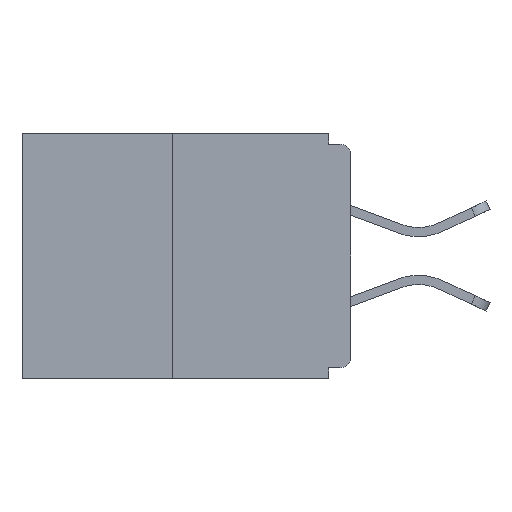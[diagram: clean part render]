
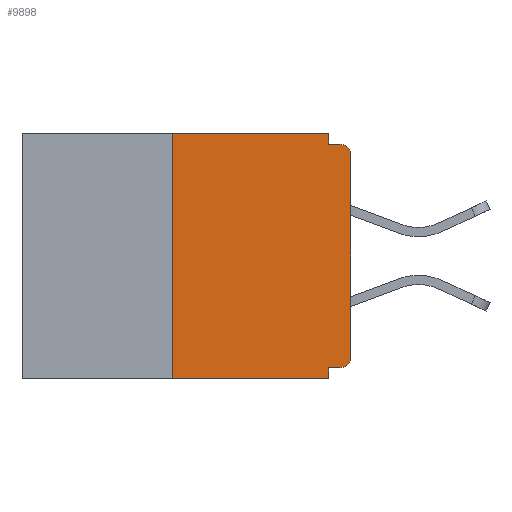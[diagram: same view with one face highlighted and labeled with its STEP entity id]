
A CAD part, left-side view. The second image highlights one B-rep face of the part: STEP entity #9898.
In plain terms, the highlighted planar face has unit normal (-1, 0, 0).
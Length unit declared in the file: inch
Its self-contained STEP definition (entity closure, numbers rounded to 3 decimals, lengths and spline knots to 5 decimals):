
#55 = DIRECTION ( 'NONE',  ( 0., 0., -1. ) ) ;
#77 = VERTEX_POINT ( 'NONE', #13116 ) ;
#89 = ORIENTED_EDGE ( 'NONE', *, *, #696, .F. ) ;
#140 = EDGE_CURVE ( 'NONE', #28373, #24476, #27689, .T. ) ;
#260 = CARTESIAN_POINT ( 'NONE',  ( 0., 0., 0. ) ) ;
#696 = EDGE_CURVE ( 'NONE', #29795, #15816, #27579, .T. ) ;
#936 = CARTESIAN_POINT ( 'NONE',  ( 0., 0.031, -0.343 ) ) ;
#1424 = CARTESIAN_POINT ( 'NONE',  ( 0., 0.015, -0.03 ) ) ;
#1528 = DIRECTION ( 'NONE',  ( 0., -1., 0. ) ) ;
#2436 = ORIENTED_EDGE ( 'NONE', *, *, #25723, .F. ) ;
#3128 = PLANE ( 'NONE',  #16647 ) ;
#3170 = CARTESIAN_POINT ( 'NONE',  ( 0., 0.031, 0. ) ) ;
#3340 = DIRECTION ( 'NONE',  ( 0., 0., -1. ) ) ;
#3561 = CARTESIAN_POINT ( 'NONE',  ( 0., 0., -0.313 ) ) ;
#3753 = CARTESIAN_POINT ( 'NONE',  ( 0., 0., -0.328 ) ) ;
#3880 = CARTESIAN_POINT ( 'NONE',  ( 0., 0., -0.03 ) ) ;
#3927 = CARTESIAN_POINT ( 'NONE',  ( 0., 0.031, 0. ) ) ;
#4766 = LINE ( 'NONE', #23429, #12398 ) ;
#4807 = ORIENTED_EDGE ( 'NONE', *, *, #20768, .T. ) ;
#4923 = VECTOR ( 'NONE', #12303, 39.37008 ) ;
#5707 = VECTOR ( 'NONE', #8784, 39.37008 ) ;
#6485 = LINE ( 'NONE', #13892, #5707 ) ;
#6752 = EDGE_CURVE ( 'NONE', #15816, #22791, #4766, .T. ) ;
#6961 = DIRECTION ( 'NONE',  ( -1., 0., 0. ) ) ;
#7391 = VERTEX_POINT ( 'NONE', #25448 ) ;
#7812 = LINE ( 'NONE', #260, #4923 ) ;
#7909 = CIRCLE ( 'NONE', #10279, 0.015 ) ;
#8032 = LINE ( 'NONE', #11750, #19474 ) ;
#8784 = DIRECTION ( 'NONE',  ( 0., 0., -1. ) ) ;
#9290 = ORIENTED_EDGE ( 'NONE', *, *, #6752, .F. ) ;
#9316 = ORIENTED_EDGE ( 'NONE', *, *, #140, .T. ) ;
#9734 = DIRECTION ( 'NONE',  ( 0., -1., 0. ) ) ;
#9898 = ADVANCED_FACE ( 'NONE', ( #25603 ), #3128, .F. ) ;
#10116 = EDGE_CURVE ( 'NONE', #22791, #7391, #23639, .T. ) ;
#10279 = AXIS2_PLACEMENT_3D ( 'NONE', #14534, #6961, #55 ) ;
#10282 = ORIENTED_EDGE ( 'NONE', *, *, #28740, .T. ) ;
#11229 = CARTESIAN_POINT ( 'NONE',  ( 0., 0.25, 0. ) ) ;
#11750 = CARTESIAN_POINT ( 'NONE',  ( 0., 0., -0.015 ) ) ;
#12006 = VECTOR ( 'NONE', #30299, 39.37008 ) ;
#12303 = DIRECTION ( 'NONE',  ( 0., 0., 1. ) ) ;
#12327 = LINE ( 'NONE', #28982, #19585 ) ;
#12398 = VECTOR ( 'NONE', #1528, 39.37008 ) ;
#12668 = EDGE_CURVE ( 'NONE', #7391, #24476, #8032, .T. ) ;
#13116 = CARTESIAN_POINT ( 'NONE',  ( 0., 0.031, -0.328 ) ) ;
#13540 = DIRECTION ( 'NONE',  ( 0., 0., -1. ) ) ;
#13892 = CARTESIAN_POINT ( 'NONE',  ( 0., 0.031, -0.343 ) ) ;
#14534 = CARTESIAN_POINT ( 'NONE',  ( 0., 0.015, -0.313 ) ) ;
#15384 = DIRECTION ( 'NONE',  ( 1., 0., 0. ) ) ;
#15688 = DIRECTION ( 'NONE',  ( -1., 0., 0. ) ) ;
#15816 = VERTEX_POINT ( 'NONE', #11229 ) ;
#16279 = VERTEX_POINT ( 'NONE', #3561 ) ;
#16340 = DIRECTION ( 'NONE',  ( 0., 1., 0. ) ) ;
#16647 = AXIS2_PLACEMENT_3D ( 'NONE', #27402, #15384, #3340 ) ;
#17050 = CARTESIAN_POINT ( 'NONE',  ( 0., 0.25, -0.343 ) ) ;
#17673 = VECTOR ( 'NONE', #16340, 39.37008 ) ;
#18310 = CARTESIAN_POINT ( 'NONE',  ( 0., 0.015, -0.015 ) ) ;
#18668 = ORIENTED_EDGE ( 'NONE', *, *, #10116, .F. ) ;
#19399 = AXIS2_PLACEMENT_3D ( 'NONE', #1424, #15688, #13540 ) ;
#19474 = VECTOR ( 'NONE', #23657, 39.37008 ) ;
#19585 = VECTOR ( 'NONE', #9734, 39.37008 ) ;
#19959 = LINE ( 'NONE', #3753, #17673 ) ;
#20010 = DIRECTION ( 'NONE',  ( 0., 0., -1. ) ) ;
#20768 = EDGE_CURVE ( 'NONE', #29795, #22190, #12327, .T. ) ;
#22190 = VERTEX_POINT ( 'NONE', #936 ) ;
#22227 = EDGE_LOOP ( 'NONE', ( #9290, #89, #4807, #25659, #2436, #26772, #10282, #9316, #24820, #18668 ) ) ;
#22791 = VERTEX_POINT ( 'NONE', #3927 ) ;
#23109 = CARTESIAN_POINT ( 'NONE',  ( 0., 0.25, 0. ) ) ;
#23429 = CARTESIAN_POINT ( 'NONE',  ( 0., 0.46, 0. ) ) ;
#23639 = LINE ( 'NONE', #3170, #28563 ) ;
#23657 = DIRECTION ( 'NONE',  ( 0., -1., 0. ) ) ;
#24476 = VERTEX_POINT ( 'NONE', #18310 ) ;
#24820 = ORIENTED_EDGE ( 'NONE', *, *, #12668, .F. ) ;
#25247 = CARTESIAN_POINT ( 'NONE',  ( 0., 0.015, -0.328 ) ) ;
#25448 = CARTESIAN_POINT ( 'NONE',  ( 0., 0.031, -0.015 ) ) ;
#25603 = FACE_OUTER_BOUND ( 'NONE', #22227, .T. ) ;
#25659 = ORIENTED_EDGE ( 'NONE', *, *, #28487, .F. ) ;
#25723 = EDGE_CURVE ( 'NONE', #31284, #77, #19959, .T. ) ;
#26772 = ORIENTED_EDGE ( 'NONE', *, *, #29206, .T. ) ;
#27402 = CARTESIAN_POINT ( 'NONE',  ( 0., 0.46, 0. ) ) ;
#27579 = LINE ( 'NONE', #23109, #12006 ) ;
#27689 = CIRCLE ( 'NONE', #19399, 0.015 ) ;
#28373 = VERTEX_POINT ( 'NONE', #3880 ) ;
#28487 = EDGE_CURVE ( 'NONE', #77, #22190, #6485, .T. ) ;
#28563 = VECTOR ( 'NONE', #20010, 39.37008 ) ;
#28740 = EDGE_CURVE ( 'NONE', #16279, #28373, #7812, .T. ) ;
#28982 = CARTESIAN_POINT ( 'NONE',  ( 0., 0.46, -0.343 ) ) ;
#29206 = EDGE_CURVE ( 'NONE', #31284, #16279, #7909, .T. ) ;
#29795 = VERTEX_POINT ( 'NONE', #17050 ) ;
#30299 = DIRECTION ( 'NONE',  ( 0., 0., 1. ) ) ;
#31284 = VERTEX_POINT ( 'NONE', #25247 ) ;
